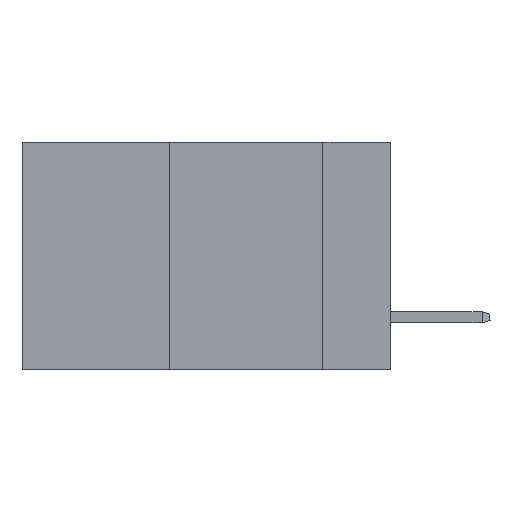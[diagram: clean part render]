
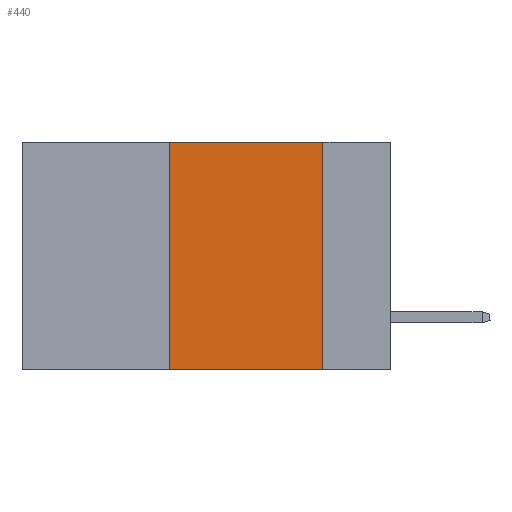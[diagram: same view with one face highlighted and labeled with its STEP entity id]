
A CAD part, left-side view. The second image highlights one B-rep face of the part: STEP entity #440.
In plain terms, the highlighted planar face has unit normal (-1, 0, 0).
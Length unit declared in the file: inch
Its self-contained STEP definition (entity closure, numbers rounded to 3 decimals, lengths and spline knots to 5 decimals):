
#440 = ADVANCED_FACE ( 'NONE', ( #15925 ), #22224, .F. ) ;
#1598 = DIRECTION ( 'NONE',  ( 1., 0., 0. ) ) ;
#2485 = VERTEX_POINT ( 'NONE', #24764 ) ;
#3023 = VECTOR ( 'NONE', #29771, 39.37008 ) ;
#3122 = ORIENTED_EDGE ( 'NONE', *, *, #25589, .F. ) ;
#3812 = DIRECTION ( 'NONE',  ( 0., 0., -1. ) ) ;
#4458 = CARTESIAN_POINT ( 'NONE',  ( 0., 0.6, -0.37 ) ) ;
#5128 = LINE ( 'NONE', #20989, #8025 ) ;
#6535 = EDGE_CURVE ( 'NONE', #7089, #2485, #26154, .T. ) ;
#7089 = VERTEX_POINT ( 'NONE', #11183 ) ;
#7479 = VERTEX_POINT ( 'NONE', #24398 ) ;
#7497 = LINE ( 'NONE', #12732, #8557 ) ;
#7783 = VERTEX_POINT ( 'NONE', #23189 ) ;
#8025 = VECTOR ( 'NONE', #11760, 39.37008 ) ;
#8557 = VECTOR ( 'NONE', #12831, 39.37008 ) ;
#11183 = CARTESIAN_POINT ( 'NONE',  ( 0., 0.36, -0.37 ) ) ;
#11760 = DIRECTION ( 'NONE',  ( 0., -1., 0. ) ) ;
#12180 = DIRECTION ( 'NONE',  ( 0., 0., 1. ) ) ;
#12732 = CARTESIAN_POINT ( 'NONE',  ( 0., 0.11, 0. ) ) ;
#12831 = DIRECTION ( 'NONE',  ( 0., 0., -1. ) ) ;
#13489 = EDGE_CURVE ( 'NONE', #7089, #7783, #14258, .T. ) ;
#13521 = VECTOR ( 'NONE', #12180, 39.37008 ) ;
#14258 = LINE ( 'NONE', #28216, #13521 ) ;
#15925 = FACE_OUTER_BOUND ( 'NONE', #27503, .T. ) ;
#16673 = AXIS2_PLACEMENT_3D ( 'NONE', #17673, #1598, #3812 ) ;
#17673 = CARTESIAN_POINT ( 'NONE',  ( 0., 0.6, 0. ) ) ;
#17805 = ORIENTED_EDGE ( 'NONE', *, *, #13489, .F. ) ;
#20212 = ORIENTED_EDGE ( 'NONE', *, *, #6535, .T. ) ;
#20989 = CARTESIAN_POINT ( 'NONE',  ( 0., 0.6, 0. ) ) ;
#22224 = PLANE ( 'NONE',  #16673 ) ;
#23189 = CARTESIAN_POINT ( 'NONE',  ( 0., 0.36, 0. ) ) ;
#24064 = EDGE_CURVE ( 'NONE', #7479, #2485, #7497, .T. ) ;
#24398 = CARTESIAN_POINT ( 'NONE',  ( 0., 0.11, 0. ) ) ;
#24764 = CARTESIAN_POINT ( 'NONE',  ( 0., 0.11, -0.37 ) ) ;
#24928 = ORIENTED_EDGE ( 'NONE', *, *, #24064, .F. ) ;
#25589 = EDGE_CURVE ( 'NONE', #7783, #7479, #5128, .T. ) ;
#26154 = LINE ( 'NONE', #4458, #3023 ) ;
#27503 = EDGE_LOOP ( 'NONE', ( #24928, #3122, #17805, #20212 ) ) ;
#28216 = CARTESIAN_POINT ( 'NONE',  ( 0., 0.36, 0. ) ) ;
#29771 = DIRECTION ( 'NONE',  ( 0., -1., 0. ) ) ;
